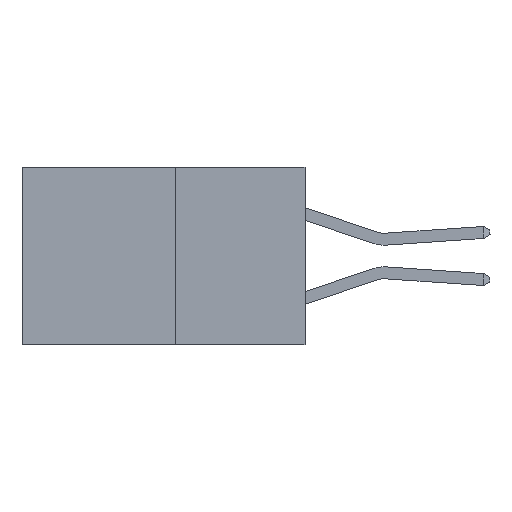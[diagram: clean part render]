
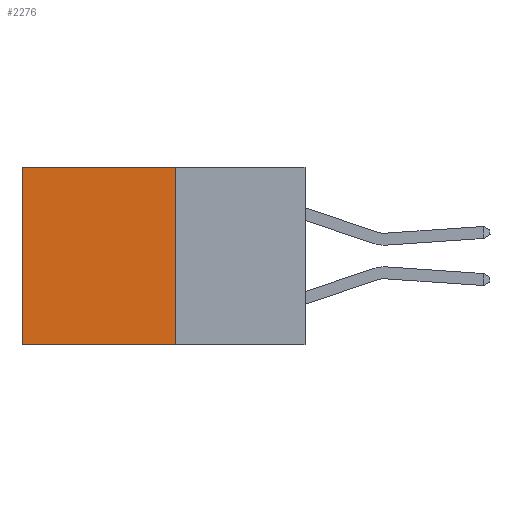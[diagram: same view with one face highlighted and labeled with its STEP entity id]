
A CAD part, left-side view. The second image highlights one B-rep face of the part: STEP entity #2276.
In plain terms, the highlighted planar face has unit normal (-1, 0, 0).
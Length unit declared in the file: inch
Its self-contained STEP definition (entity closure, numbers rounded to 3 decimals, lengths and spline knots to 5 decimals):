
#718 = VERTEX_POINT ( 'NONE', #3150 ) ;
#738 = DIRECTION ( 'NONE',  ( 0., 1., 0. ) ) ;
#766 = CARTESIAN_POINT ( 'NONE',  ( 0.277, 0.59, -0.37 ) ) ;
#1192 = DIRECTION ( 'NONE',  ( 0., 0., -1. ) ) ;
#1222 = CARTESIAN_POINT ( 'NONE',  ( 0.277, 0.27, -0.37 ) ) ;
#1819 = DIRECTION ( 'NONE',  ( 0., 0., -1. ) ) ;
#1940 = ORIENTED_EDGE ( 'NONE', *, *, #3333, .F. ) ;
#1963 = AXIS2_PLACEMENT_3D ( 'NONE', #4032, #3513, #3448 ) ;
#2276 = ADVANCED_FACE ( 'NONE', ( #6007 ), #3561, .F. ) ;
#2362 = CARTESIAN_POINT ( 'NONE',  ( 0.277, 0.27, 0. ) ) ;
#2540 = VECTOR ( 'NONE', #1819, 39.37008 ) ;
#2866 = LINE ( 'NONE', #766, #2540 ) ;
#3150 = CARTESIAN_POINT ( 'NONE',  ( 0.277, 0.27, -0.37 ) ) ;
#3333 = EDGE_CURVE ( 'NONE', #718, #3581, #11388, .T. ) ;
#3448 = DIRECTION ( 'NONE',  ( 0., 0., -1. ) ) ;
#3513 = DIRECTION ( 'NONE',  ( 1., 0., 0. ) ) ;
#3561 = PLANE ( 'NONE',  #1963 ) ;
#3581 = VERTEX_POINT ( 'NONE', #9149 ) ;
#3729 = EDGE_LOOP ( 'NONE', ( #6674, #1940, #4686, #7230 ) ) ;
#4021 = EDGE_CURVE ( 'NONE', #5494, #718, #6314, .T. ) ;
#4032 = CARTESIAN_POINT ( 'NONE',  ( 0.277, 0.27, -0.37 ) ) ;
#4686 = ORIENTED_EDGE ( 'NONE', *, *, #4021, .F. ) ;
#4826 = CARTESIAN_POINT ( 'NONE',  ( 0.277, 0.27, 0. ) ) ;
#4900 = DIRECTION ( 'NONE',  ( 0., 1., 0. ) ) ;
#5030 = CARTESIAN_POINT ( 'NONE',  ( 0.277, 0.27, -0.37 ) ) ;
#5494 = VERTEX_POINT ( 'NONE', #2362 ) ;
#6007 = FACE_OUTER_BOUND ( 'NONE', #3729, .T. ) ;
#6314 = LINE ( 'NONE', #1222, #10729 ) ;
#6674 = ORIENTED_EDGE ( 'NONE', *, *, #9386, .T. ) ;
#7113 = CARTESIAN_POINT ( 'NONE',  ( 0.277, 0.59, 0. ) ) ;
#7230 = ORIENTED_EDGE ( 'NONE', *, *, #7855, .T. ) ;
#7306 = VERTEX_POINT ( 'NONE', #7113 ) ;
#7855 = EDGE_CURVE ( 'NONE', #5494, #7306, #8030, .T. ) ;
#8030 = LINE ( 'NONE', #4826, #10161 ) ;
#9149 = CARTESIAN_POINT ( 'NONE',  ( 0.277, 0.59, -0.37 ) ) ;
#9246 = VECTOR ( 'NONE', #4900, 39.37008 ) ;
#9386 = EDGE_CURVE ( 'NONE', #7306, #3581, #2866, .T. ) ;
#10161 = VECTOR ( 'NONE', #738, 39.37008 ) ;
#10729 = VECTOR ( 'NONE', #1192, 39.37008 ) ;
#11388 = LINE ( 'NONE', #5030, #9246 ) ;
